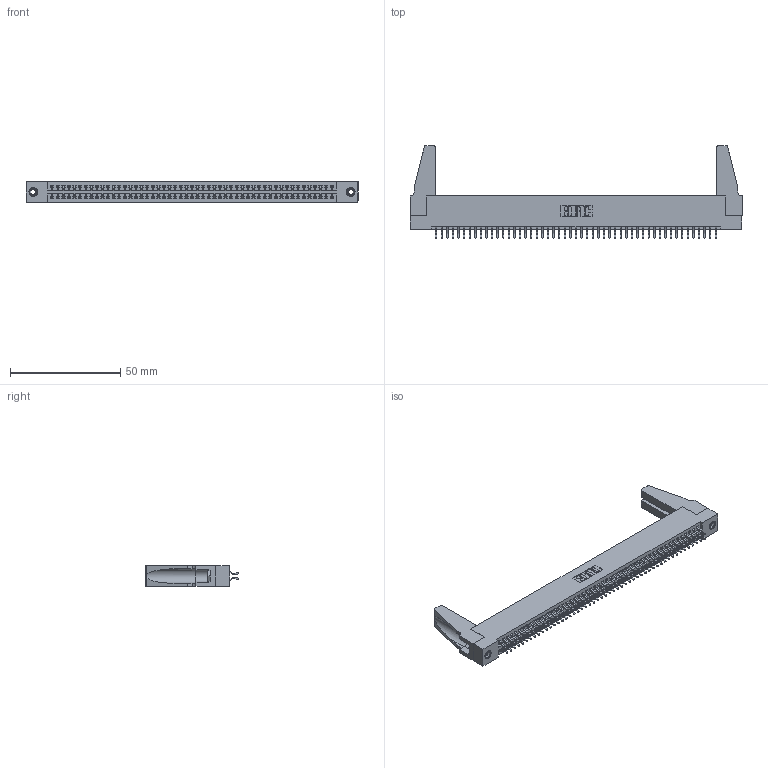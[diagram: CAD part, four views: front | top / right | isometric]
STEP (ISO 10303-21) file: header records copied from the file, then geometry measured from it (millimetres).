
FILE_DESCRIPTION (( 'STEP AP203' ), '1' );
FILE_NAME ('345-102-556-288.STEP', '2019-11-03T09:00:16', ( '' ), ( '' ), 'SwSTEP 2.0', 'SolidWorks 2016', '' );
FILE_SCHEMA (( 'CONFIG_CONTROL_DESIGN' ));
Length unit declared in the file: inch
Products named in the file (5): 345 Part_Flush Mounting Lugs - 0.156 Dia-TH; 345-102-556-288; 345-292-001_556 Tail; 345-220-078_345-220-088; 345-250-001_345-250-001-102
Assembly tree (107 placements, depth 2):
  345-102-556-288
    345 Part_Flush Mounting Lugs - 0.156 Dia-TH
    345-292-001_556 Tail  x102
    345-250-001_345-250-001-102  x2
    345-220-078_345-220-088  x2
Bounding box: 150.77 x 42.1 x 9.4 mm (x, y, z)
Volume: 17978.3 mm3; surface area: 24974.5 mm2
Topology: 107 solids, 107 shells, 5962 faces, 17689 edges, 11646 vertices
Faces by surface type: plane 3926, cylinder 2020, cone 12, torus 4
Entity records: 41172 total; most frequent: CARTESIAN_POINT 6902, ORIENTED_EDGE 6784, DIRECTION 6068, EDGE_CURVE 3392, LINE 3006, VECTOR 3006, VERTEX_POINT 2254, AXIS2_PLACEMENT_3D 1531
